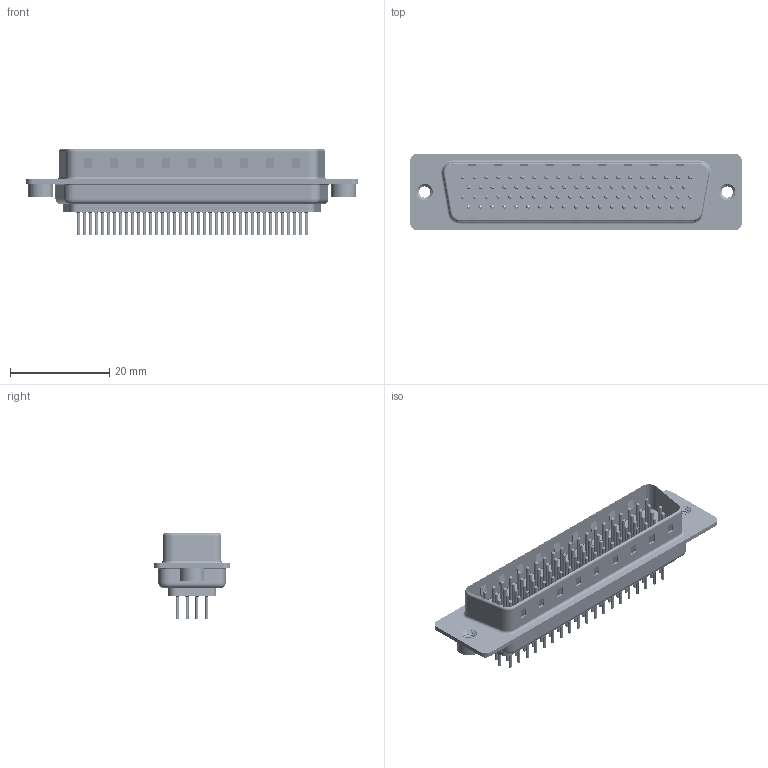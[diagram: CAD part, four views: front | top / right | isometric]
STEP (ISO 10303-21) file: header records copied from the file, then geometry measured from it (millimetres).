
FILE_DESCRIPTION (( 'STEP AP203' ), '1' );
FILE_NAME ('637-078-230-262.STEP', '2020-07-18T05:17:02', ( '' ), ( '' ), 'SwSTEP 2.0', 'SolidWorks 2020', '' );
FILE_SCHEMA (( 'CONFIG_CONTROL_DESIGN' ));
Length unit declared in the file: millimetre
Products named in the file (9): 637 Contact Row 2_30; 637 Contact Row 78_30; 637 Contact Row 1_30; 637 Housing_78 Contacts; 637 Shell Front_78 Contacts; 637-078-230-262; 637 Shell Rear_78 Contacts; 637 Contact Row 3_30; 637 4-40 Threaded Rivet
Assembly tree (83 placements, depth 2):
  637-078-230-262
    637 Housing_78 Contacts
    637 Shell Front_78 Contacts
    637 Shell Rear_78 Contacts
    637 Contact Row 1_30  x19
    637 Contact Row 2_30  x20
    637 Contact Row 3_30  x19
    637 Contact Row 78_30  x20
    637 4-40 Threaded Rivet  x2
Bounding box: 67 x 15.4 x 17.25 mm (x, y, z)
Volume: 4336 mm3; surface area: 15864.6 mm2
Topology: 83 solids, 83 shells, 8212 faces, 21727 edges, 13380 vertices
Faces by surface type: cylinder 3027, torus 2312, plane 2075, cone 792, bspline 6
Entity records: 46674 total; most frequent: CARTESIAN_POINT 9549, DIRECTION 7790, ORIENTED_EDGE 6672, EDGE_CURVE 3336, AXIS2_PLACEMENT_3D 3183, VERTEX_POINT 2146, EDGE_LOOP 1742, CIRCLE 1729
